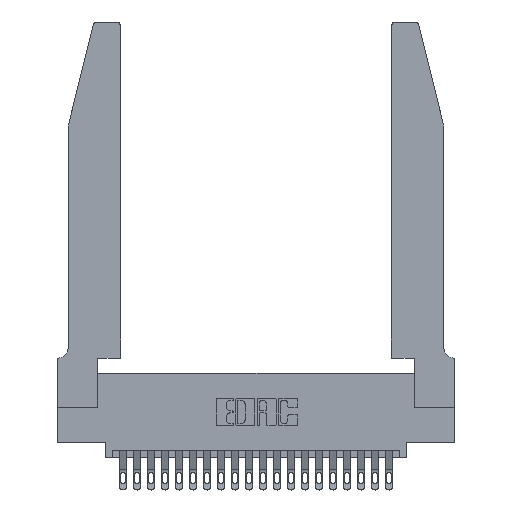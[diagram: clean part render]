
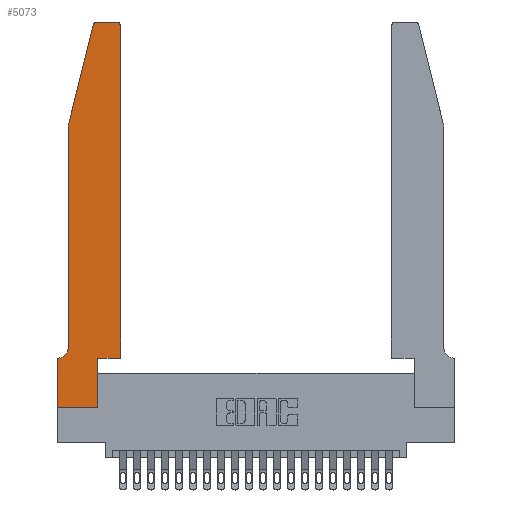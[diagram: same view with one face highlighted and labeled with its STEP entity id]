
A CAD part, top view. The second image highlights one B-rep face of the part: STEP entity #5073.
In plain terms, the highlighted planar face has unit normal (0, 0, 1).
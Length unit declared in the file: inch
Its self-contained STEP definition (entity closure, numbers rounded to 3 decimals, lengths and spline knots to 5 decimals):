
#43 = DIRECTION ( 'NONE',  ( 0., 0., -1. ) ) ;
#99 = DIRECTION ( 'NONE',  ( -1., 0., 0. ) ) ;
#192 = VERTEX_POINT ( 'NONE', #18782 ) ;
#207 = ORIENTED_EDGE ( 'NONE', *, *, #14436, .T. ) ;
#544 = CARTESIAN_POINT ( 'NONE',  ( 0.284, 2.75, 0.37 ) ) ;
#797 = DIRECTION ( 'NONE',  ( 1., 0., 0. ) ) ;
#1232 = LINE ( 'NONE', #13869, #3546 ) ;
#1234 = CARTESIAN_POINT ( 'NONE',  ( 0., 0.35, 0.37 ) ) ;
#1379 = DIRECTION ( 'NONE',  ( 0., 0., 1. ) ) ;
#1693 = ORIENTED_EDGE ( 'NONE', *, *, #11044, .T. ) ;
#2331 = EDGE_CURVE ( 'NONE', #12897, #23577, #15164, .T. ) ;
#2405 = AXIS2_PLACEMENT_3D ( 'NONE', #14924, #21996, #11059 ) ;
#2573 = EDGE_LOOP ( 'NONE', ( #20879, #4170, #1693, #10722, #9672, #19831, #16983, #6300, #4693, #12200, #207, #11964 ) ) ;
#2641 = LINE ( 'NONE', #22864, #20215 ) ;
#3148 = CARTESIAN_POINT ( 'NONE',  ( 0., 0.35, 0.37 ) ) ;
#3335 = DIRECTION ( 'NONE',  ( 0., -1., 0. ) ) ;
#3546 = VECTOR ( 'NONE', #20057, 39.37008 ) ;
#3860 = CARTESIAN_POINT ( 'NONE',  ( 0.2865, 0.35, 0.37 ) ) ;
#4170 = ORIENTED_EDGE ( 'NONE', *, *, #20068, .T. ) ;
#4261 = LINE ( 'NONE', #19848, #18371 ) ;
#4693 = ORIENTED_EDGE ( 'NONE', *, *, #9656, .T. ) ;
#4723 = EDGE_CURVE ( 'NONE', #15113, #13401, #8138, .T. ) ;
#4877 = LINE ( 'NONE', #7635, #5724 ) ;
#5073 = ADVANCED_FACE ( 'NONE', ( #13581 ), #21498, .T. ) ;
#5108 = CARTESIAN_POINT ( 'NONE',  ( 0.0755, 2., 0.37 ) ) ;
#5405 = LINE ( 'NONE', #19114, #21783 ) ;
#5508 = CARTESIAN_POINT ( 'NONE',  ( 0.0055, 0.42, 0.37 ) ) ;
#5637 = VERTEX_POINT ( 'NONE', #5108 ) ;
#5724 = VECTOR ( 'NONE', #16632, 39.37008 ) ;
#5905 = CARTESIAN_POINT ( 'NONE',  ( 0.4205, 2.75, 0.37 ) ) ;
#6300 = ORIENTED_EDGE ( 'NONE', *, *, #2331, .T. ) ;
#6617 = AXIS2_PLACEMENT_3D ( 'NONE', #5508, #43, #9357 ) ;
#7247 = DIRECTION ( 'NONE',  ( 0., 1., 0. ) ) ;
#7635 = CARTESIAN_POINT ( 'NONE',  ( 0.0755, 2., 0.37 ) ) ;
#7680 = CARTESIAN_POINT ( 'NONE',  ( 0.2865, 0.35, 0.37 ) ) ;
#7692 = CARTESIAN_POINT ( 'NONE',  ( 0., 0., 0.37 ) ) ;
#7864 = EDGE_CURVE ( 'NONE', #9400, #13658, #5405, .T. ) ;
#8138 = CIRCLE ( 'NONE', #2405, 0.03 ) ;
#8497 = CARTESIAN_POINT ( 'NONE',  ( 0.4505, 0.35, 0.37 ) ) ;
#8653 = EDGE_CURVE ( 'NONE', #19501, #19078, #2641, .T. ) ;
#8948 = VECTOR ( 'NONE', #99, 39.37008 ) ;
#9357 = DIRECTION ( 'NONE',  ( -1., 0., 0. ) ) ;
#9400 = VERTEX_POINT ( 'NONE', #23145 ) ;
#9493 = CARTESIAN_POINT ( 'NONE',  ( 0.284, 2.72, 0.37 ) ) ;
#9656 = EDGE_CURVE ( 'NONE', #23577, #19501, #20745, .T. ) ;
#9672 = ORIENTED_EDGE ( 'NONE', *, *, #17617, .T. ) ;
#9726 = CARTESIAN_POINT ( 'NONE',  ( 0.4505, 2.72, 0.37 ) ) ;
#10007 = CARTESIAN_POINT ( 'NONE',  ( 0., 0., 0.37 ) ) ;
#10640 = DIRECTION ( 'NONE',  ( 1., 0., 0. ) ) ;
#10722 = ORIENTED_EDGE ( 'NONE', *, *, #21345, .T. ) ;
#11044 = EDGE_CURVE ( 'NONE', #23214, #5637, #20436, .T. ) ;
#11059 = DIRECTION ( 'NONE',  ( 1., 0., 0. ) ) ;
#11964 = ORIENTED_EDGE ( 'NONE', *, *, #4723, .T. ) ;
#12200 = ORIENTED_EDGE ( 'NONE', *, *, #8653, .T. ) ;
#12723 = VECTOR ( 'NONE', #7247, 39.37008 ) ;
#12879 = CARTESIAN_POINT ( 'NONE',  ( 0.25487, 2.72718, 0.37 ) ) ;
#12897 = VERTEX_POINT ( 'NONE', #7692 ) ;
#13139 = DIRECTION ( 'NONE',  ( 0., 0., 1. ) ) ;
#13401 = VERTEX_POINT ( 'NONE', #5905 ) ;
#13581 = FACE_OUTER_BOUND ( 'NONE', #2573, .T. ) ;
#13658 = VERTEX_POINT ( 'NONE', #1234 ) ;
#13869 = CARTESIAN_POINT ( 'NONE',  ( 0.4505, 0.35, 0.37 ) ) ;
#14436 = EDGE_CURVE ( 'NONE', #19078, #15113, #1232, .T. ) ;
#14924 = CARTESIAN_POINT ( 'NONE',  ( 0.4205, 2.72, 0.37 ) ) ;
#15113 = VERTEX_POINT ( 'NONE', #9726 ) ;
#15164 = LINE ( 'NONE', #10007, #21778 ) ;
#16486 = DIRECTION ( 'NONE',  ( 1., 0., 0. ) ) ;
#16633 = VERTEX_POINT ( 'NONE', #544 ) ;
#16632 = DIRECTION ( 'NONE',  ( 0., -1., 0. ) ) ;
#16719 = CARTESIAN_POINT ( 'NONE',  ( 0.2605, 2.75, 0.37 ) ) ;
#16969 = VECTOR ( 'NONE', #17143, 39.37008 ) ;
#16983 = ORIENTED_EDGE ( 'NONE', *, *, #21711, .T. ) ;
#17010 = CIRCLE ( 'NONE', #18633, 0.03 ) ;
#17143 = DIRECTION ( 'NONE',  ( -0.239, -0.971, 0. ) ) ;
#17617 = EDGE_CURVE ( 'NONE', #192, #9400, #22271, .T. ) ;
#18303 = CARTESIAN_POINT ( 'NONE',  ( 0.2865, 0., 0.37 ) ) ;
#18371 = VECTOR ( 'NONE', #3335, 39.37008 ) ;
#18633 = AXIS2_PLACEMENT_3D ( 'NONE', #9493, #13139, #16486 ) ;
#18782 = CARTESIAN_POINT ( 'NONE',  ( 0.0755, 0.42, 0.37 ) ) ;
#19078 = VERTEX_POINT ( 'NONE', #8497 ) ;
#19114 = CARTESIAN_POINT ( 'NONE',  ( 0.0755, 0.35, 0.37 ) ) ;
#19376 = DIRECTION ( 'NONE',  ( 1., 0., 0. ) ) ;
#19501 = VERTEX_POINT ( 'NONE', #7680 ) ;
#19831 = ORIENTED_EDGE ( 'NONE', *, *, #7864, .T. ) ;
#19848 = CARTESIAN_POINT ( 'NONE',  ( 0., 0., 0.37 ) ) ;
#20057 = DIRECTION ( 'NONE',  ( 0., 1., 0. ) ) ;
#20068 = EDGE_CURVE ( 'NONE', #16633, #23214, #17010, .T. ) ;
#20110 = EDGE_CURVE ( 'NONE', #13401, #16633, #23354, .T. ) ;
#20215 = VECTOR ( 'NONE', #19376, 39.37008 ) ;
#20436 = LINE ( 'NONE', #22630, #16969 ) ;
#20745 = LINE ( 'NONE', #3860, #12723 ) ;
#20879 = ORIENTED_EDGE ( 'NONE', *, *, #20110, .T. ) ;
#21266 = DIRECTION ( 'NONE',  ( -1., 0., 0. ) ) ;
#21345 = EDGE_CURVE ( 'NONE', #5637, #192, #4877, .T. ) ;
#21498 = PLANE ( 'NONE',  #22641 ) ;
#21711 = EDGE_CURVE ( 'NONE', #13658, #12897, #4261, .T. ) ;
#21778 = VECTOR ( 'NONE', #797, 39.37008 ) ;
#21783 = VECTOR ( 'NONE', #21266, 39.37008 ) ;
#21996 = DIRECTION ( 'NONE',  ( 0., 0., 1. ) ) ;
#22271 = CIRCLE ( 'NONE', #6617, 0.07 ) ;
#22630 = CARTESIAN_POINT ( 'NONE',  ( 0.0755, 2., 0.37 ) ) ;
#22641 = AXIS2_PLACEMENT_3D ( 'NONE', #3148, #1379, #10640 ) ;
#22864 = CARTESIAN_POINT ( 'NONE',  ( 0.4505, 0.35, 0.37 ) ) ;
#23145 = CARTESIAN_POINT ( 'NONE',  ( 0.0055, 0.35, 0.37 ) ) ;
#23214 = VERTEX_POINT ( 'NONE', #12879 ) ;
#23354 = LINE ( 'NONE', #16719, #8948 ) ;
#23577 = VERTEX_POINT ( 'NONE', #18303 ) ;
